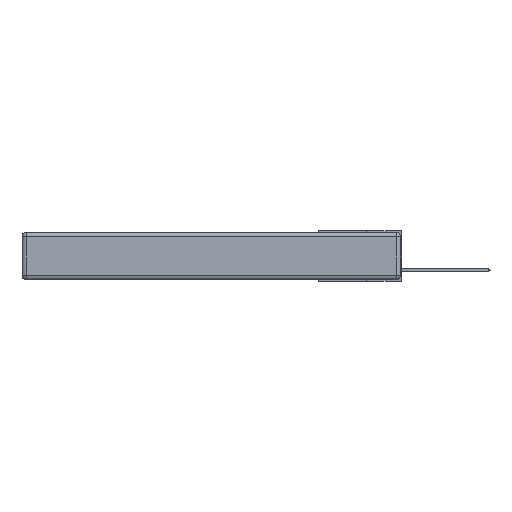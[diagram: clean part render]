
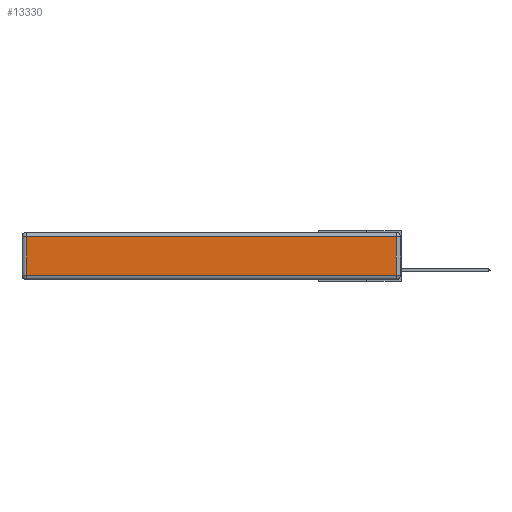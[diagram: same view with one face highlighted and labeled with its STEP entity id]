
A CAD part, left-side view. The second image highlights one B-rep face of the part: STEP entity #13330.
In plain terms, the highlighted planar face has unit normal (-1, 0, 0).
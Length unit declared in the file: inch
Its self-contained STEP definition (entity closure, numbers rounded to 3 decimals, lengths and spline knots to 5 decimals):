
#58 = EDGE_LOOP ( 'NONE', ( #12374, #7504, #768, #10427 ) ) ;
#280 = CARTESIAN_POINT ( 'NONE',  ( 0., 0., -0.343 ) ) ;
#768 = ORIENTED_EDGE ( 'NONE', *, *, #9346, .T. ) ;
#778 = VECTOR ( 'NONE', #7822, 39.37008 ) ;
#931 = VERTEX_POINT ( 'NONE', #12952 ) ;
#1152 = CARTESIAN_POINT ( 'NONE',  ( 0., 0., -0.313 ) ) ;
#1612 = EDGE_CURVE ( 'NONE', #5306, #4590, #2244, .T. ) ;
#1758 = DIRECTION ( 'NONE',  ( -1., 0., 0. ) ) ;
#2132 = CARTESIAN_POINT ( 'NONE',  ( 0., 2.75, -0.03 ) ) ;
#2244 = LINE ( 'NONE', #11682, #778 ) ;
#3851 = DIRECTION ( 'NONE',  ( 0., -1., 0. ) ) ;
#4501 = VECTOR ( 'NONE', #3851, 39.37008 ) ;
#4590 = VERTEX_POINT ( 'NONE', #14495 ) ;
#4967 = EDGE_CURVE ( 'NONE', #931, #7070, #6099, .T. ) ;
#5306 = VERTEX_POINT ( 'NONE', #13590 ) ;
#5955 = CARTESIAN_POINT ( 'NONE',  ( 0., 0.03, -0.343 ) ) ;
#6099 = LINE ( 'NONE', #5955, #10702 ) ;
#7000 = DIRECTION ( 'NONE',  ( 0., 0., 1. ) ) ;
#7070 = VERTEX_POINT ( 'NONE', #9848 ) ;
#7413 = DIRECTION ( 'NONE',  ( 0., 0., 1. ) ) ;
#7504 = ORIENTED_EDGE ( 'NONE', *, *, #4967, .T. ) ;
#7822 = DIRECTION ( 'NONE',  ( 0., 0., -1. ) ) ;
#8357 = PLANE ( 'NONE',  #15948 ) ;
#8449 = LINE ( 'NONE', #2132, #11585 ) ;
#9346 = EDGE_CURVE ( 'NONE', #7070, #5306, #8449, .T. ) ;
#9848 = CARTESIAN_POINT ( 'NONE',  ( 0., 0.03, -0.03 ) ) ;
#10427 = ORIENTED_EDGE ( 'NONE', *, *, #1612, .T. ) ;
#10702 = VECTOR ( 'NONE', #7413, 39.37008 ) ;
#11437 = DIRECTION ( 'NONE',  ( 0., 1., 0. ) ) ;
#11585 = VECTOR ( 'NONE', #11437, 39.37008 ) ;
#11682 = CARTESIAN_POINT ( 'NONE',  ( 0., 2.72, -0.343 ) ) ;
#12305 = LINE ( 'NONE', #1152, #4501 ) ;
#12374 = ORIENTED_EDGE ( 'NONE', *, *, #14972, .T. ) ;
#12952 = CARTESIAN_POINT ( 'NONE',  ( 0., 0.03, -0.313 ) ) ;
#13330 = ADVANCED_FACE ( 'NONE', ( #13607 ), #8357, .T. ) ;
#13590 = CARTESIAN_POINT ( 'NONE',  ( 0., 2.72, -0.03 ) ) ;
#13607 = FACE_OUTER_BOUND ( 'NONE', #58, .T. ) ;
#14495 = CARTESIAN_POINT ( 'NONE',  ( 0., 2.72, -0.313 ) ) ;
#14972 = EDGE_CURVE ( 'NONE', #4590, #931, #12305, .T. ) ;
#15948 = AXIS2_PLACEMENT_3D ( 'NONE', #280, #1758, #7000 ) ;
